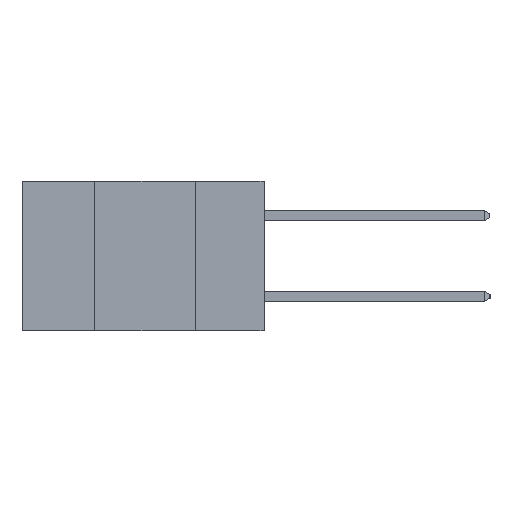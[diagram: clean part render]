
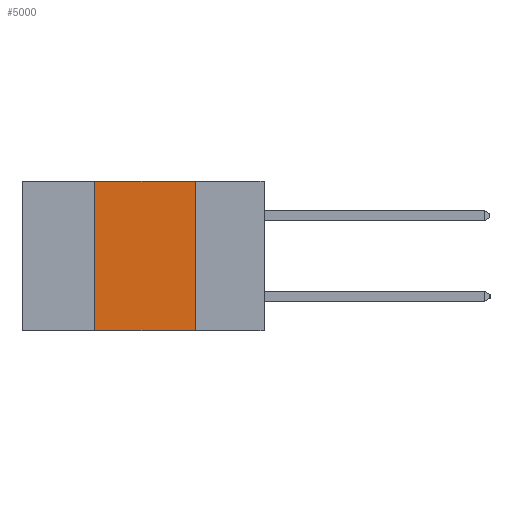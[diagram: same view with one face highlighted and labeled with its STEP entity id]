
A CAD part, left-side view. The second image highlights one B-rep face of the part: STEP entity #5000.
In plain terms, the highlighted planar face has unit normal (-1, 0, 0).
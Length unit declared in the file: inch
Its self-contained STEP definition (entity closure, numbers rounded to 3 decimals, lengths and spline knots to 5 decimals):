
#69 = ORIENTED_EDGE ( 'NONE', *, *, #6505, .T. ) ;
#506 = VERTEX_POINT ( 'NONE', #5364 ) ;
#917 = LINE ( 'NONE', #5885, #9966 ) ;
#976 = VERTEX_POINT ( 'NONE', #10492 ) ;
#1027 = VERTEX_POINT ( 'NONE', #4448 ) ;
#1054 = LINE ( 'NONE', #9624, #8104 ) ;
#2763 = VECTOR ( 'NONE', #4876, 39.37008 ) ;
#2899 = FACE_OUTER_BOUND ( 'NONE', #3011, .T. ) ;
#3011 = EDGE_LOOP ( 'NONE', ( #8906, #11091, #9183, #69 ) ) ;
#3113 = VERTEX_POINT ( 'NONE', #11244 ) ;
#3115 = CARTESIAN_POINT ( 'NONE',  ( 0., 0.42, -0.37 ) ) ;
#3120 = DIRECTION ( 'NONE',  ( 0., 0., -1. ) ) ;
#3191 = DIRECTION ( 'NONE',  ( 1., 0., 0. ) ) ;
#3262 = CARTESIAN_POINT ( 'NONE',  ( 0., 0.6, 0. ) ) ;
#3511 = DIRECTION ( 'NONE',  ( 0., -1., 0. ) ) ;
#3638 = PLANE ( 'NONE',  #5519 ) ;
#4448 = CARTESIAN_POINT ( 'NONE',  ( 0., 0.42, 0. ) ) ;
#4488 = EDGE_CURVE ( 'NONE', #3113, #506, #917, .T. ) ;
#4494 = VECTOR ( 'NONE', #3511, 39.37008 ) ;
#4761 = EDGE_CURVE ( 'NONE', #1027, #3113, #1054, .T. ) ;
#4876 = DIRECTION ( 'NONE',  ( 0., 0., 1. ) ) ;
#5000 = ADVANCED_FACE ( 'NONE', ( #2899 ), #3638, .F. ) ;
#5156 = EDGE_CURVE ( 'NONE', #976, #1027, #9828, .T. ) ;
#5364 = CARTESIAN_POINT ( 'NONE',  ( 0., 0.17, -0.37 ) ) ;
#5519 = AXIS2_PLACEMENT_3D ( 'NONE', #3262, #3191, #3120 ) ;
#5885 = CARTESIAN_POINT ( 'NONE',  ( 0., 0.17, -0.37 ) ) ;
#6505 = EDGE_CURVE ( 'NONE', #976, #506, #9518, .T. ) ;
#8104 = VECTOR ( 'NONE', #10171, 39.37008 ) ;
#8906 = ORIENTED_EDGE ( 'NONE', *, *, #4488, .F. ) ;
#9183 = ORIENTED_EDGE ( 'NONE', *, *, #5156, .F. ) ;
#9518 = LINE ( 'NONE', #9730, #4494 ) ;
#9624 = CARTESIAN_POINT ( 'NONE',  ( 0., 0.6, 0. ) ) ;
#9730 = CARTESIAN_POINT ( 'NONE',  ( 0., 0.6, -0.37 ) ) ;
#9828 = LINE ( 'NONE', #3115, #2763 ) ;
#9966 = VECTOR ( 'NONE', #10471, 39.37008 ) ;
#10171 = DIRECTION ( 'NONE',  ( 0., -1., 0. ) ) ;
#10471 = DIRECTION ( 'NONE',  ( 0., 0., -1. ) ) ;
#10492 = CARTESIAN_POINT ( 'NONE',  ( 0., 0.42, -0.37 ) ) ;
#11091 = ORIENTED_EDGE ( 'NONE', *, *, #4761, .F. ) ;
#11244 = CARTESIAN_POINT ( 'NONE',  ( 0., 0.17, 0. ) ) ;
